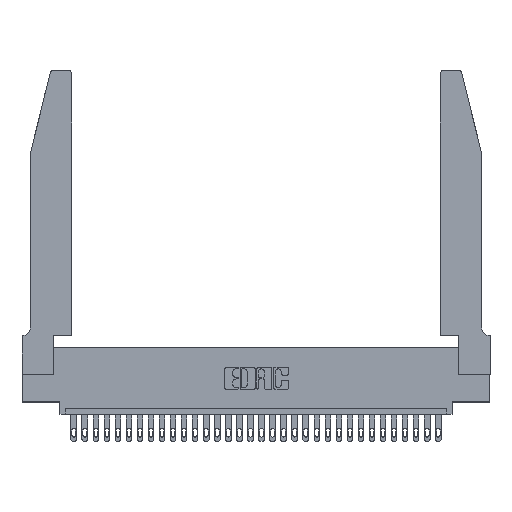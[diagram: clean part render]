
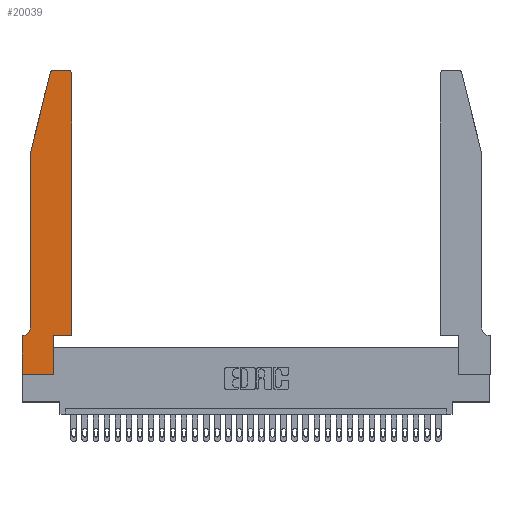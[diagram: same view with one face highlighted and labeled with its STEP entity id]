
A CAD part, top view. The second image highlights one B-rep face of the part: STEP entity #20039.
In plain terms, the highlighted planar face has unit normal (0, 0, 1).
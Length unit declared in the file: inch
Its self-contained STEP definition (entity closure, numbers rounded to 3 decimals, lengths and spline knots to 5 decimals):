
#576 = DIRECTION ( 'NONE',  ( -0.239, -0.971, 0. ) ) ;
#893 = ORIENTED_EDGE ( 'NONE', *, *, #11201, .T. ) ;
#945 = LINE ( 'NONE', #19782, #4387 ) ;
#1305 = AXIS2_PLACEMENT_3D ( 'NONE', #7311, #21996, #16927 ) ;
#1594 = AXIS2_PLACEMENT_3D ( 'NONE', #23969, #4076, #16542 ) ;
#1800 = CARTESIAN_POINT ( 'NONE',  ( 0.0055, 0.42, 0.37 ) ) ;
#2540 = LINE ( 'NONE', #7192, #4093 ) ;
#2576 = EDGE_CURVE ( 'NONE', #9829, #17683, #14650, .T. ) ;
#2886 = LINE ( 'NONE', #29833, #11331 ) ;
#2954 = VECTOR ( 'NONE', #4077, 39.37008 ) ;
#3179 = LINE ( 'NONE', #19142, #26441 ) ;
#3628 = VERTEX_POINT ( 'NONE', #7273 ) ;
#3816 = EDGE_CURVE ( 'NONE', #17683, #30445, #22633, .T. ) ;
#4076 = DIRECTION ( 'NONE',  ( 0., 0., 1. ) ) ;
#4077 = DIRECTION ( 'NONE',  ( -1., 0., 0. ) ) ;
#4093 = VECTOR ( 'NONE', #576, 39.37008 ) ;
#4160 = ORIENTED_EDGE ( 'NONE', *, *, #4576, .T. ) ;
#4346 = EDGE_CURVE ( 'NONE', #22614, #14972, #14626, .T. ) ;
#4387 = VECTOR ( 'NONE', #15868, 39.37008 ) ;
#4395 = EDGE_CURVE ( 'NONE', #30445, #3628, #3179, .T. ) ;
#4499 = DIRECTION ( 'NONE',  ( 0., -1., 0. ) ) ;
#4576 = EDGE_CURVE ( 'NONE', #28430, #22614, #945, .T. ) ;
#4795 = AXIS2_PLACEMENT_3D ( 'NONE', #18806, #29188, #19620 ) ;
#5802 = EDGE_CURVE ( 'NONE', #3628, #8644, #21814, .T. ) ;
#6122 = CARTESIAN_POINT ( 'NONE',  ( 0.4505, 0.35, 0.37 ) ) ;
#6248 = CARTESIAN_POINT ( 'NONE',  ( 0.4505, 2.72, 0.37 ) ) ;
#6593 = DIRECTION ( 'NONE',  ( -1., 0., 0. ) ) ;
#6785 = ORIENTED_EDGE ( 'NONE', *, *, #4395, .T. ) ;
#7110 = PLANE ( 'NONE',  #1305 ) ;
#7192 = CARTESIAN_POINT ( 'NONE',  ( 0.0755, 2., 0.37 ) ) ;
#7248 = CIRCLE ( 'NONE', #1594, 0.03 ) ;
#7273 = CARTESIAN_POINT ( 'NONE',  ( 0.2865, 0.35, 0.37 ) ) ;
#7311 = CARTESIAN_POINT ( 'NONE',  ( 0., 0.35, 0.37 ) ) ;
#7778 = LINE ( 'NONE', #6122, #20346 ) ;
#8159 = VECTOR ( 'NONE', #4499, 39.37008 ) ;
#8644 = VERTEX_POINT ( 'NONE', #25446 ) ;
#8836 = ORIENTED_EDGE ( 'NONE', *, *, #23849, .T. ) ;
#8848 = CARTESIAN_POINT ( 'NONE',  ( 0.0755, 0.42, 0.37 ) ) ;
#8916 = EDGE_CURVE ( 'NONE', #30803, #28430, #2540, .T. ) ;
#9068 = CARTESIAN_POINT ( 'NONE',  ( 0., 0., 0.37 ) ) ;
#9829 = VERTEX_POINT ( 'NONE', #31146 ) ;
#11170 = CARTESIAN_POINT ( 'NONE',  ( 0., 0., 0.37 ) ) ;
#11201 = EDGE_CURVE ( 'NONE', #8644, #12455, #7778, .T. ) ;
#11331 = VECTOR ( 'NONE', #15390, 39.37008 ) ;
#12156 = CARTESIAN_POINT ( 'NONE',  ( 0.284, 2.75, 0.37 ) ) ;
#12455 = VERTEX_POINT ( 'NONE', #6248 ) ;
#12646 = ORIENTED_EDGE ( 'NONE', *, *, #4346, .T. ) ;
#12981 = ORIENTED_EDGE ( 'NONE', *, *, #20481, .T. ) ;
#13341 = CIRCLE ( 'NONE', #4795, 0.03 ) ;
#13540 = CARTESIAN_POINT ( 'NONE',  ( 0.4205, 2.75, 0.37 ) ) ;
#13757 = ORIENTED_EDGE ( 'NONE', *, *, #14689, .T. ) ;
#13764 = FACE_OUTER_BOUND ( 'NONE', #19811, .T. ) ;
#14626 = CIRCLE ( 'NONE', #26087, 0.07 ) ;
#14650 = LINE ( 'NONE', #9068, #8159 ) ;
#14689 = EDGE_CURVE ( 'NONE', #21311, #15714, #26228, .T. ) ;
#14972 = VERTEX_POINT ( 'NONE', #18081 ) ;
#15327 = VECTOR ( 'NONE', #28087, 39.37008 ) ;
#15390 = DIRECTION ( 'NONE',  ( -1., 0., 0. ) ) ;
#15714 = VERTEX_POINT ( 'NONE', #12156 ) ;
#15868 = DIRECTION ( 'NONE',  ( 0., -1., 0. ) ) ;
#16266 = EDGE_CURVE ( 'NONE', #14972, #9829, #2886, .T. ) ;
#16542 = DIRECTION ( 'NONE',  ( 1., 0., 0. ) ) ;
#16842 = CARTESIAN_POINT ( 'NONE',  ( 0.0755, 2., 0.37 ) ) ;
#16927 = DIRECTION ( 'NONE',  ( 1., 0., 0. ) ) ;
#17683 = VERTEX_POINT ( 'NONE', #11170 ) ;
#18081 = CARTESIAN_POINT ( 'NONE',  ( 0.0055, 0.35, 0.37 ) ) ;
#18669 = CARTESIAN_POINT ( 'NONE',  ( 0.2605, 2.75, 0.37 ) ) ;
#18806 = CARTESIAN_POINT ( 'NONE',  ( 0.4205, 2.72, 0.37 ) ) ;
#18931 = ORIENTED_EDGE ( 'NONE', *, *, #5802, .T. ) ;
#19142 = CARTESIAN_POINT ( 'NONE',  ( 0.2865, 0.35, 0.37 ) ) ;
#19620 = DIRECTION ( 'NONE',  ( 1., 0., 0. ) ) ;
#19782 = CARTESIAN_POINT ( 'NONE',  ( 0.0755, 2., 0.37 ) ) ;
#19811 = EDGE_LOOP ( 'NONE', ( #13757, #8836, #30098, #4160, #12646, #24645, #27676, #30749, #6785, #18931, #893, #12981 ) ) ;
#20039 = ADVANCED_FACE ( 'NONE', ( #13764 ), #7110, .T. ) ;
#20346 = VECTOR ( 'NONE', #22360, 39.37008 ) ;
#20481 = EDGE_CURVE ( 'NONE', #12455, #21311, #13341, .T. ) ;
#21171 = DIRECTION ( 'NONE',  ( 0., 1., 0. ) ) ;
#21311 = VERTEX_POINT ( 'NONE', #13540 ) ;
#21814 = LINE ( 'NONE', #30847, #15327 ) ;
#21996 = DIRECTION ( 'NONE',  ( 0., 0., 1. ) ) ;
#22360 = DIRECTION ( 'NONE',  ( 0., 1., 0. ) ) ;
#22614 = VERTEX_POINT ( 'NONE', #8848 ) ;
#22633 = LINE ( 'NONE', #22672, #30647 ) ;
#22672 = CARTESIAN_POINT ( 'NONE',  ( 0., 0., 0.37 ) ) ;
#23520 = CARTESIAN_POINT ( 'NONE',  ( 0.25487, 2.72718, 0.37 ) ) ;
#23849 = EDGE_CURVE ( 'NONE', #15714, #30803, #7248, .T. ) ;
#23918 = DIRECTION ( 'NONE',  ( 0., 0., -1. ) ) ;
#23969 = CARTESIAN_POINT ( 'NONE',  ( 0.284, 2.72, 0.37 ) ) ;
#24466 = CARTESIAN_POINT ( 'NONE',  ( 0.2865, 0., 0.37 ) ) ;
#24645 = ORIENTED_EDGE ( 'NONE', *, *, #16266, .T. ) ;
#25446 = CARTESIAN_POINT ( 'NONE',  ( 0.4505, 0.35, 0.37 ) ) ;
#26087 = AXIS2_PLACEMENT_3D ( 'NONE', #1800, #23918, #6593 ) ;
#26228 = LINE ( 'NONE', #18669, #2954 ) ;
#26441 = VECTOR ( 'NONE', #21171, 39.37008 ) ;
#27673 = DIRECTION ( 'NONE',  ( 1., 0., 0. ) ) ;
#27676 = ORIENTED_EDGE ( 'NONE', *, *, #2576, .T. ) ;
#28087 = DIRECTION ( 'NONE',  ( 1., 0., 0. ) ) ;
#28430 = VERTEX_POINT ( 'NONE', #16842 ) ;
#29188 = DIRECTION ( 'NONE',  ( 0., 0., 1. ) ) ;
#29833 = CARTESIAN_POINT ( 'NONE',  ( 0.0755, 0.35, 0.37 ) ) ;
#30098 = ORIENTED_EDGE ( 'NONE', *, *, #8916, .T. ) ;
#30445 = VERTEX_POINT ( 'NONE', #24466 ) ;
#30647 = VECTOR ( 'NONE', #27673, 39.37008 ) ;
#30749 = ORIENTED_EDGE ( 'NONE', *, *, #3816, .T. ) ;
#30803 = VERTEX_POINT ( 'NONE', #23520 ) ;
#30847 = CARTESIAN_POINT ( 'NONE',  ( 0.4505, 0.35, 0.37 ) ) ;
#31146 = CARTESIAN_POINT ( 'NONE',  ( 0., 0.35, 0.37 ) ) ;
